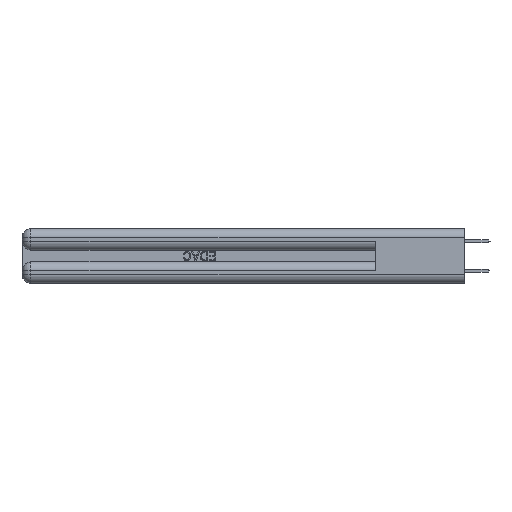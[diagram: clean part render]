
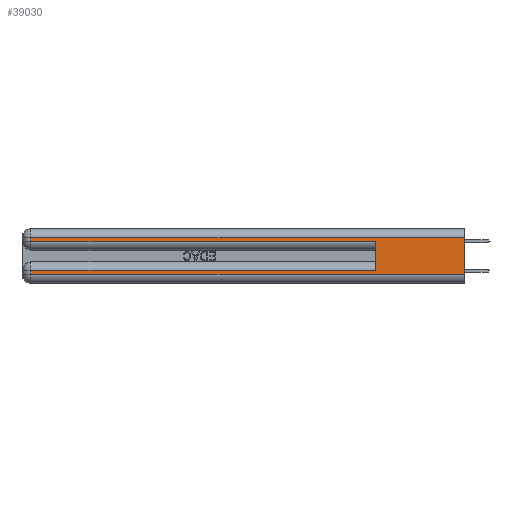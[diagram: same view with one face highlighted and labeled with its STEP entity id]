
A CAD part, left-side view. The second image highlights one B-rep face of the part: STEP entity #39030.
In plain terms, the highlighted planar face has unit normal (-1, 0, 0).
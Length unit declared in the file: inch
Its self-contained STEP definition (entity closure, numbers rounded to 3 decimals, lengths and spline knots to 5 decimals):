
#1128 = CARTESIAN_POINT ( 'NONE',  ( 0., 2.94, 0.06 ) ) ;
#1208 = CARTESIAN_POINT ( 'NONE',  ( 0., 0., 0.06 ) ) ;
#2408 = CARTESIAN_POINT ( 'NONE',  ( 0., 2.94, 0.31 ) ) ;
#3215 = ORIENTED_EDGE ( 'NONE', *, *, #23618, .T. ) ;
#3563 = DIRECTION ( 'NONE',  ( 0., 0., -1. ) ) ;
#3735 = DIRECTION ( 'NONE',  ( 0., 1., 0. ) ) ;
#3754 = EDGE_CURVE ( 'NONE', #39649, #18320, #28175, .T. ) ;
#3936 = LINE ( 'NONE', #40615, #5081 ) ;
#3958 = VECTOR ( 'NONE', #23320, 39.37008 ) ;
#4265 = VECTOR ( 'NONE', #34742, 39.37008 ) ;
#5081 = VECTOR ( 'NONE', #44360, 39.37008 ) ;
#5457 = CARTESIAN_POINT ( 'NONE',  ( 0., 0., 0.31 ) ) ;
#6026 = DIRECTION ( 'NONE',  ( 1., 0., 0. ) ) ;
#7391 = LINE ( 'NONE', #33486, #16097 ) ;
#7796 = VERTEX_POINT ( 'NONE', #19182 ) ;
#9645 = VECTOR ( 'NONE', #42179, 39.37008 ) ;
#10227 = ORIENTED_EDGE ( 'NONE', *, *, #35101, .F. ) ;
#10423 = ORIENTED_EDGE ( 'NONE', *, *, #3754, .T. ) ;
#10822 = FACE_OUTER_BOUND ( 'NONE', #24356, .T. ) ;
#11385 = EDGE_CURVE ( 'NONE', #7796, #26675, #23962, .T. ) ;
#11970 = CARTESIAN_POINT ( 'NONE',  ( 0., 0., 0.285 ) ) ;
#13169 = EDGE_CURVE ( 'NONE', #42617, #39649, #22848, .T. ) ;
#13303 = PLANE ( 'NONE',  #25064 ) ;
#15288 = VECTOR ( 'NONE', #3563, 39.37008 ) ;
#15536 = CARTESIAN_POINT ( 'NONE',  ( 0., 2.94, 0.37 ) ) ;
#16097 = VECTOR ( 'NONE', #25859, 39.37008 ) ;
#16638 = EDGE_CURVE ( 'NONE', #18320, #26675, #24812, .T. ) ;
#18172 = VERTEX_POINT ( 'NONE', #1208 ) ;
#18320 = VERTEX_POINT ( 'NONE', #46249 ) ;
#19182 = CARTESIAN_POINT ( 'NONE',  ( 0., 0.6, 0.085 ) ) ;
#19520 = LINE ( 'NONE', #27328, #9645 ) ;
#22366 = CARTESIAN_POINT ( 'NONE',  ( 0., 2.94, 0.085 ) ) ;
#22848 = LINE ( 'NONE', #40639, #42536 ) ;
#22888 = ORIENTED_EDGE ( 'NONE', *, *, #13169, .T. ) ;
#23320 = DIRECTION ( 'NONE',  ( 0., -1., 0. ) ) ;
#23618 = EDGE_CURVE ( 'NONE', #44188, #44365, #3936, .T. ) ;
#23962 = LINE ( 'NONE', #31051, #4265 ) ;
#24257 = EDGE_CURVE ( 'NONE', #7796, #44188, #7391, .T. ) ;
#24356 = EDGE_LOOP ( 'NONE', ( #10227, #22888, #10423, #42480, #30155, #45972, #3215, #29253 ) ) ;
#24812 = LINE ( 'NONE', #11970, #3958 ) ;
#25064 = AXIS2_PLACEMENT_3D ( 'NONE', #28289, #6026, #32002 ) ;
#25766 = CARTESIAN_POINT ( 'NONE',  ( 0., 0., 0.37 ) ) ;
#25859 = DIRECTION ( 'NONE',  ( 0., 1., 0. ) ) ;
#26675 = VERTEX_POINT ( 'NONE', #27432 ) ;
#27328 = CARTESIAN_POINT ( 'NONE',  ( 0., 0., 0.06 ) ) ;
#27432 = CARTESIAN_POINT ( 'NONE',  ( 0., 0.6, 0.285 ) ) ;
#28175 = LINE ( 'NONE', #15536, #47856 ) ;
#28289 = CARTESIAN_POINT ( 'NONE',  ( 0., 0., 0.37 ) ) ;
#29253 = ORIENTED_EDGE ( 'NONE', *, *, #43192, .T. ) ;
#30155 = ORIENTED_EDGE ( 'NONE', *, *, #11385, .F. ) ;
#31051 = CARTESIAN_POINT ( 'NONE',  ( 0., 0.6, 0.145 ) ) ;
#32002 = DIRECTION ( 'NONE',  ( 0., 0., -1. ) ) ;
#33486 = CARTESIAN_POINT ( 'NONE',  ( 0., 0., 0.085 ) ) ;
#34742 = DIRECTION ( 'NONE',  ( 0., 0., 1. ) ) ;
#35101 = EDGE_CURVE ( 'NONE', #42617, #18172, #36201, .T. ) ;
#36201 = LINE ( 'NONE', #25766, #15288 ) ;
#37752 = DIRECTION ( 'NONE',  ( 0., 0., -1. ) ) ;
#39030 = ADVANCED_FACE ( 'NONE', ( #10822 ), #13303, .F. ) ;
#39649 = VERTEX_POINT ( 'NONE', #2408 ) ;
#40615 = CARTESIAN_POINT ( 'NONE',  ( 0., 2.94, 0.37 ) ) ;
#40639 = CARTESIAN_POINT ( 'NONE',  ( 0., 0., 0.31 ) ) ;
#42179 = DIRECTION ( 'NONE',  ( 0., -1., 0. ) ) ;
#42480 = ORIENTED_EDGE ( 'NONE', *, *, #16638, .T. ) ;
#42536 = VECTOR ( 'NONE', #3735, 39.37008 ) ;
#42617 = VERTEX_POINT ( 'NONE', #5457 ) ;
#43192 = EDGE_CURVE ( 'NONE', #44365, #18172, #19520, .T. ) ;
#44188 = VERTEX_POINT ( 'NONE', #22366 ) ;
#44360 = DIRECTION ( 'NONE',  ( 0., 0., -1. ) ) ;
#44365 = VERTEX_POINT ( 'NONE', #1128 ) ;
#45972 = ORIENTED_EDGE ( 'NONE', *, *, #24257, .T. ) ;
#46249 = CARTESIAN_POINT ( 'NONE',  ( 0., 2.94, 0.285 ) ) ;
#47856 = VECTOR ( 'NONE', #37752, 39.37008 ) ;
